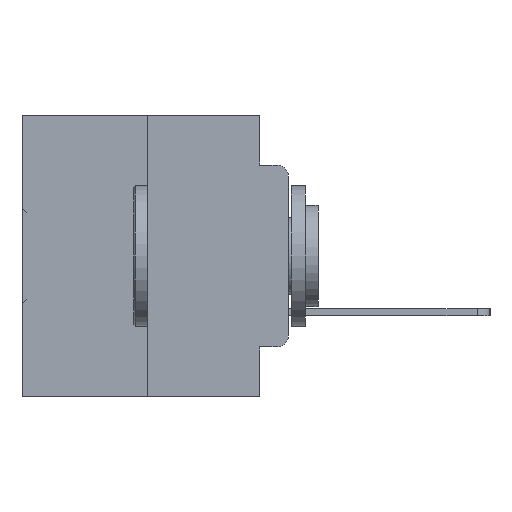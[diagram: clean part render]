
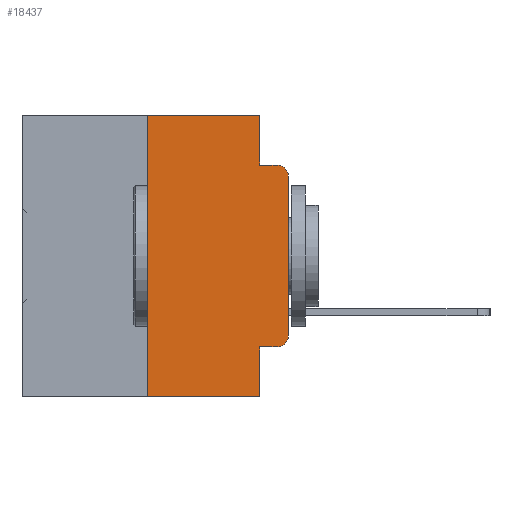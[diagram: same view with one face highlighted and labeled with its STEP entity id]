
A CAD part, left-side view. The second image highlights one B-rep face of the part: STEP entity #18437.
In plain terms, the highlighted planar face has unit normal (-1, 0, 0).
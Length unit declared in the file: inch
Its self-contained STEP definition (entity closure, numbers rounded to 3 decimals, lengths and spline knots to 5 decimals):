
#62 = CIRCLE ( 'NONE', #26508, 0.02 ) ;
#130 = EDGE_CURVE ( 'NONE', #3386, #5152, #18939, .T. ) ;
#438 = CARTESIAN_POINT ( 'NONE',  ( 0., 0.02, -0.3915 ) ) ;
#1048 = VERTEX_POINT ( 'NONE', #28634 ) ;
#1992 = VECTOR ( 'NONE', #34886, 39.37008 ) ;
#2005 = EDGE_CURVE ( 'NONE', #14691, #34123, #30746, .T. ) ;
#3264 = DIRECTION ( 'NONE',  ( 0., 0., -1. ) ) ;
#3386 = VERTEX_POINT ( 'NONE', #25125 ) ;
#5152 = VERTEX_POINT ( 'NONE', #13086 ) ;
#5242 = ORIENTED_EDGE ( 'NONE', *, *, #24022, .T. ) ;
#6002 = ORIENTED_EDGE ( 'NONE', *, *, #9529, .F. ) ;
#6108 = ORIENTED_EDGE ( 'NONE', *, *, #11327, .F. ) ;
#6436 = CARTESIAN_POINT ( 'NONE',  ( 0., 0., 0. ) ) ;
#7042 = ORIENTED_EDGE ( 'NONE', *, *, #13122, .T. ) ;
#8452 = CARTESIAN_POINT ( 'NONE',  ( 0., 0.473, 0. ) ) ;
#8876 = CARTESIAN_POINT ( 'NONE',  ( 0., 0.02, -0.1085 ) ) ;
#9207 = DIRECTION ( 'NONE',  ( 0., 0., 1. ) ) ;
#9529 = EDGE_CURVE ( 'NONE', #25200, #13043, #19277, .T. ) ;
#10365 = LINE ( 'NONE', #15090, #31132 ) ;
#10459 = EDGE_CURVE ( 'NONE', #14691, #5152, #10365, .T. ) ;
#11067 = VERTEX_POINT ( 'NONE', #28484 ) ;
#11131 = DIRECTION ( 'NONE',  ( 1., 0., 0. ) ) ;
#11327 = EDGE_CURVE ( 'NONE', #13043, #28415, #31059, .T. ) ;
#11575 = DIRECTION ( 'NONE',  ( 0., 0., -1. ) ) ;
#12439 = LINE ( 'NONE', #21966, #18732 ) ;
#13043 = VERTEX_POINT ( 'NONE', #27388 ) ;
#13086 = CARTESIAN_POINT ( 'NONE',  ( 0., 0.051, -0.5 ) ) ;
#13122 = EDGE_CURVE ( 'NONE', #1048, #28415, #33868, .T. ) ;
#13173 = CARTESIAN_POINT ( 'NONE',  ( 0., 0.02, -0.0885 ) ) ;
#13244 = CARTESIAN_POINT ( 'NONE',  ( 0., 0.051, -0.0885 ) ) ;
#13570 = FACE_OUTER_BOUND ( 'NONE', #35218, .T. ) ;
#14079 = LINE ( 'NONE', #21277, #27732 ) ;
#14691 = VERTEX_POINT ( 'NONE', #31480 ) ;
#14710 = DIRECTION ( 'NONE',  ( 0., 0., 1. ) ) ;
#15090 = CARTESIAN_POINT ( 'NONE',  ( 0., 0.473, -0.5 ) ) ;
#17400 = EDGE_CURVE ( 'NONE', #3386, #22421, #14079, .T. ) ;
#18199 = AXIS2_PLACEMENT_3D ( 'NONE', #8876, #27856, #11575 ) ;
#18437 = ADVANCED_FACE ( 'NONE', ( #13570 ), #24650, .F. ) ;
#18732 = VECTOR ( 'NONE', #32797, 39.37008 ) ;
#18939 = LINE ( 'NONE', #19832, #32557 ) ;
#19277 = LINE ( 'NONE', #32555, #25745 ) ;
#19591 = DIRECTION ( 'NONE',  ( -1., 0., 0. ) ) ;
#19832 = CARTESIAN_POINT ( 'NONE',  ( 0., 0.051, 0. ) ) ;
#20573 = AXIS2_PLACEMENT_3D ( 'NONE', #8452, #11131, #30112 ) ;
#20686 = CARTESIAN_POINT ( 'NONE',  ( 0., 0.25, 0. ) ) ;
#20986 = ORIENTED_EDGE ( 'NONE', *, *, #34434, .T. ) ;
#21277 = CARTESIAN_POINT ( 'NONE',  ( 0., 0.051, -0.4115 ) ) ;
#21383 = ORIENTED_EDGE ( 'NONE', *, *, #10459, .T. ) ;
#21756 = VECTOR ( 'NONE', #9207, 39.37008 ) ;
#21862 = ORIENTED_EDGE ( 'NONE', *, *, #17400, .T. ) ;
#21966 = CARTESIAN_POINT ( 'NONE',  ( 0., 0.473, 0. ) ) ;
#22146 = ORIENTED_EDGE ( 'NONE', *, *, #130, .F. ) ;
#22372 = CARTESIAN_POINT ( 'NONE',  ( 0., 0.25, 0. ) ) ;
#22421 = VERTEX_POINT ( 'NONE', #24799 ) ;
#23856 = EDGE_CURVE ( 'NONE', #34123, #25200, #12439, .T. ) ;
#24022 = EDGE_CURVE ( 'NONE', #11067, #1048, #35230, .T. ) ;
#24050 = DIRECTION ( 'NONE',  ( 0., -1., 0. ) ) ;
#24601 = ORIENTED_EDGE ( 'NONE', *, *, #2005, .F. ) ;
#24650 = PLANE ( 'NONE',  #20573 ) ;
#24799 = CARTESIAN_POINT ( 'NONE',  ( 0., 0.02, -0.4115 ) ) ;
#25125 = CARTESIAN_POINT ( 'NONE',  ( 0., 0.051, -0.4115 ) ) ;
#25200 = VERTEX_POINT ( 'NONE', #33615 ) ;
#25745 = VECTOR ( 'NONE', #29863, 39.37008 ) ;
#26508 = AXIS2_PLACEMENT_3D ( 'NONE', #438, #19591, #3264 ) ;
#27311 = VECTOR ( 'NONE', #14710, 39.37008 ) ;
#27388 = CARTESIAN_POINT ( 'NONE',  ( 0., 0.051, -0.0885 ) ) ;
#27409 = DIRECTION ( 'NONE',  ( 0., 0., -1. ) ) ;
#27732 = VECTOR ( 'NONE', #24050, 39.37008 ) ;
#27856 = DIRECTION ( 'NONE',  ( -1., 0., 0. ) ) ;
#28415 = VERTEX_POINT ( 'NONE', #13173 ) ;
#28484 = CARTESIAN_POINT ( 'NONE',  ( 0., 0., -0.3915 ) ) ;
#28536 = DIRECTION ( 'NONE',  ( 0., -1., 0. ) ) ;
#28634 = CARTESIAN_POINT ( 'NONE',  ( 0., 0., -0.1085 ) ) ;
#29863 = DIRECTION ( 'NONE',  ( 0., 0., -1. ) ) ;
#30112 = DIRECTION ( 'NONE',  ( 0., 0., -1. ) ) ;
#30224 = ORIENTED_EDGE ( 'NONE', *, *, #23856, .F. ) ;
#30746 = LINE ( 'NONE', #22372, #21756 ) ;
#31059 = LINE ( 'NONE', #13244, #1992 ) ;
#31132 = VECTOR ( 'NONE', #28536, 39.37008 ) ;
#31480 = CARTESIAN_POINT ( 'NONE',  ( 0., 0.25, -0.5 ) ) ;
#32555 = CARTESIAN_POINT ( 'NONE',  ( 0., 0.051, 0. ) ) ;
#32557 = VECTOR ( 'NONE', #27409, 39.37008 ) ;
#32797 = DIRECTION ( 'NONE',  ( 0., -1., 0. ) ) ;
#33615 = CARTESIAN_POINT ( 'NONE',  ( 0., 0.051, 0. ) ) ;
#33868 = CIRCLE ( 'NONE', #18199, 0.02 ) ;
#34123 = VERTEX_POINT ( 'NONE', #20686 ) ;
#34434 = EDGE_CURVE ( 'NONE', #22421, #11067, #62, .T. ) ;
#34886 = DIRECTION ( 'NONE',  ( 0., -1., 0. ) ) ;
#35218 = EDGE_LOOP ( 'NONE', ( #5242, #7042, #6108, #6002, #30224, #24601, #21383, #22146, #21862, #20986 ) ) ;
#35230 = LINE ( 'NONE', #6436, #27311 ) ;
